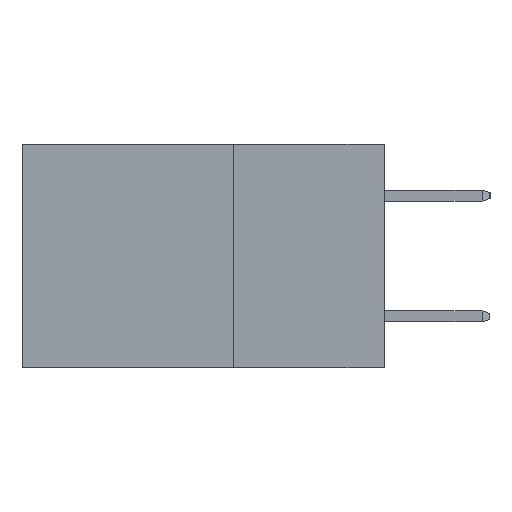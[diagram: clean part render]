
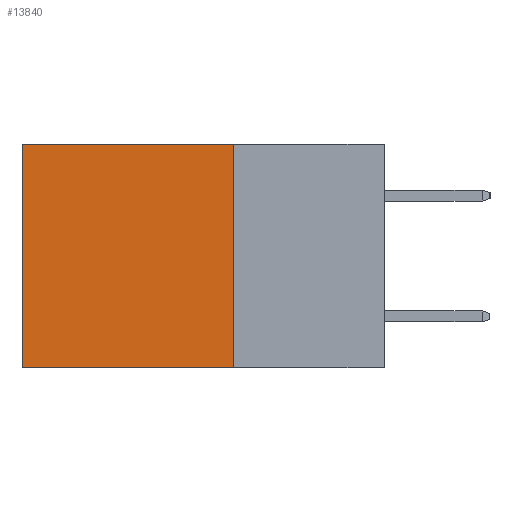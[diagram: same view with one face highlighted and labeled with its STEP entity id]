
A CAD part, left-side view. The second image highlights one B-rep face of the part: STEP entity #13840.
In plain terms, the highlighted planar face has unit normal (-1, 0, 0).
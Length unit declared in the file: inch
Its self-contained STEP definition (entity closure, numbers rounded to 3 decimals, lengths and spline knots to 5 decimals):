
#695 = VERTEX_POINT ( 'NONE', #8274 ) ;
#902 = LINE ( 'NONE', #12249, #11133 ) ;
#994 = EDGE_LOOP ( 'NONE', ( #8667, #5253, #8851, #9308 ) ) ;
#1250 = VERTEX_POINT ( 'NONE', #14361 ) ;
#1909 = CARTESIAN_POINT ( 'NONE',  ( 0.298, 0.25, 0. ) ) ;
#3109 = DIRECTION ( 'NONE',  ( 0., 0., -1. ) ) ;
#3259 = DIRECTION ( 'NONE',  ( 0., 1., 0. ) ) ;
#3658 = AXIS2_PLACEMENT_3D ( 'NONE', #1909, #10230, #3109 ) ;
#3721 = FACE_OUTER_BOUND ( 'NONE', #994, .T. ) ;
#4147 = EDGE_CURVE ( 'NONE', #9407, #1250, #13166, .T. ) ;
#4558 = EDGE_CURVE ( 'NONE', #12623, #1250, #8071, .T. ) ;
#4801 = LINE ( 'NONE', #9491, #13784 ) ;
#4871 = DIRECTION ( 'NONE',  ( 0., 1., 0. ) ) ;
#4888 = CARTESIAN_POINT ( 'NONE',  ( 0.298, 0.6, 0. ) ) ;
#5253 = ORIENTED_EDGE ( 'NONE', *, *, #4558, .F. ) ;
#6717 = EDGE_CURVE ( 'NONE', #695, #9407, #902, .T. ) ;
#7961 = EDGE_CURVE ( 'NONE', #695, #12623, #4801, .T. ) ;
#8071 = LINE ( 'NONE', #14728, #13539 ) ;
#8274 = CARTESIAN_POINT ( 'NONE',  ( 0.298, 0.25, 0. ) ) ;
#8667 = ORIENTED_EDGE ( 'NONE', *, *, #4147, .T. ) ;
#8851 = ORIENTED_EDGE ( 'NONE', *, *, #7961, .F. ) ;
#9308 = ORIENTED_EDGE ( 'NONE', *, *, #6717, .T. ) ;
#9407 = VERTEX_POINT ( 'NONE', #4888 ) ;
#9491 = CARTESIAN_POINT ( 'NONE',  ( 0.298, 0.25, 0. ) ) ;
#10132 = VECTOR ( 'NONE', #12945, 39.37008 ) ;
#10230 = DIRECTION ( 'NONE',  ( 1., 0., 0. ) ) ;
#11133 = VECTOR ( 'NONE', #4871, 39.37008 ) ;
#12069 = CARTESIAN_POINT ( 'NONE',  ( 0.298, 0.6, 0. ) ) ;
#12249 = CARTESIAN_POINT ( 'NONE',  ( 0.298, 0.25, 0. ) ) ;
#12623 = VERTEX_POINT ( 'NONE', #14812 ) ;
#12945 = DIRECTION ( 'NONE',  ( 0., 0., -1. ) ) ;
#13166 = LINE ( 'NONE', #12069, #10132 ) ;
#13539 = VECTOR ( 'NONE', #3259, 39.37008 ) ;
#13784 = VECTOR ( 'NONE', #15213, 39.37008 ) ;
#13840 = ADVANCED_FACE ( 'NONE', ( #3721 ), #14779, .F. ) ;
#14361 = CARTESIAN_POINT ( 'NONE',  ( 0.298, 0.6, -0.37 ) ) ;
#14728 = CARTESIAN_POINT ( 'NONE',  ( 0.298, 0.25, -0.37 ) ) ;
#14779 = PLANE ( 'NONE',  #3658 ) ;
#14812 = CARTESIAN_POINT ( 'NONE',  ( 0.298, 0.25, -0.37 ) ) ;
#15213 = DIRECTION ( 'NONE',  ( 0., 0., -1. ) ) ;
